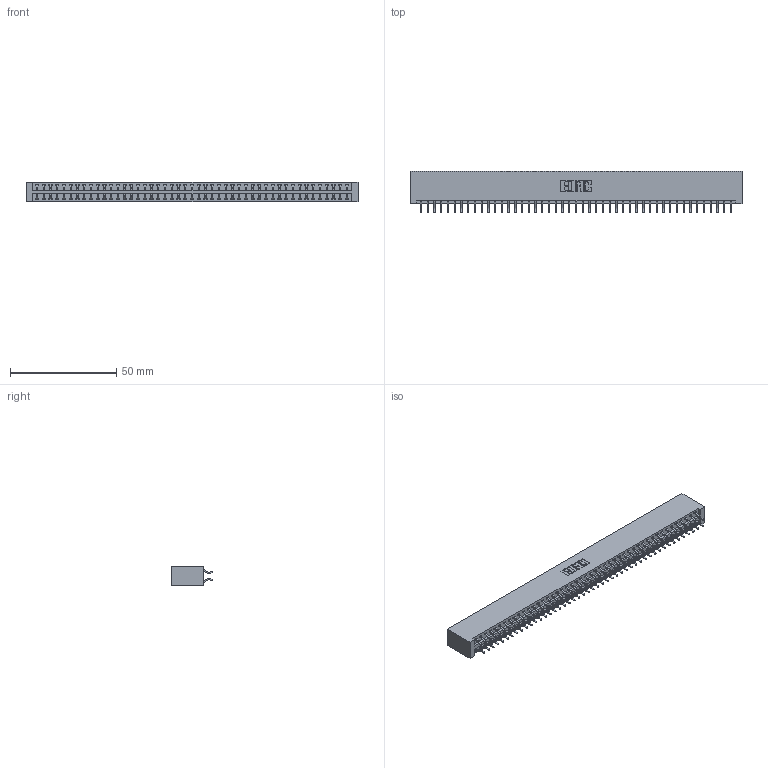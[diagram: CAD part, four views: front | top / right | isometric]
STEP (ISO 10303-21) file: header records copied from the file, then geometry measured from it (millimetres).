
FILE_DESCRIPTION (( 'STEP AP203' ), '1' );
FILE_NAME ('396-094-556-201.STEP', '2019-10-31T03:36:12', ( '' ), ( '' ), 'SwSTEP 2.0', 'SolidWorks 2016', '' );
FILE_SCHEMA (( 'CONFIG_CONTROL_DESIGN' ));
Length unit declared in the file: inch
Products named in the file (3): 345-292-001_556 Tail; 346 Part_No Mounting Lugs; 396-094-556-201
Assembly tree (95 placements, depth 2):
  396-094-556-201
    346 Part_No Mounting Lugs
    345-292-001_556 Tail  x94
Bounding box: 156.46 x 19.57 x 9.4 mm (x, y, z)
Volume: 15865.6 mm3; surface area: 21962.8 mm2
Topology: 95 solids, 95 shells, 5566 faces, 16567 edges, 10918 vertices
Faces by surface type: plane 3738, cylinder 1828
Entity records: 29943 total; most frequent: CARTESIAN_POINT 4940, ORIENTED_EDGE 4862, DIRECTION 4387, EDGE_CURVE 2431, VECTOR 2111, LINE 2111, VERTEX_POINT 1618, AXIS2_PLACEMENT_3D 1138
